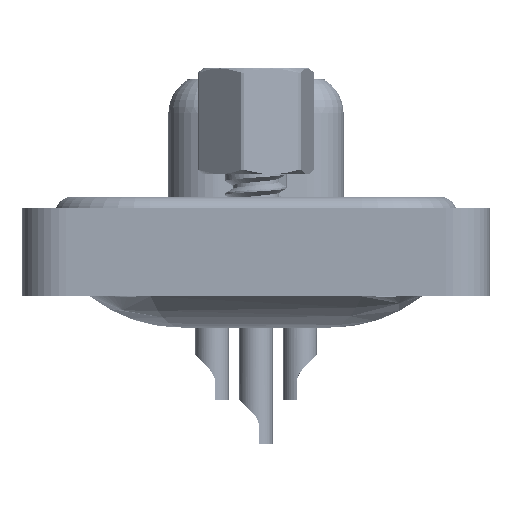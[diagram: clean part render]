
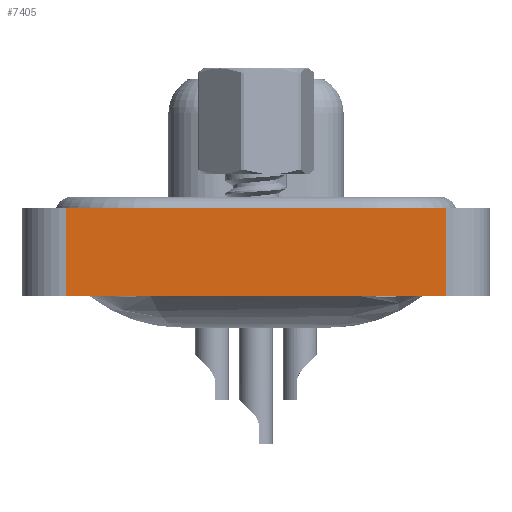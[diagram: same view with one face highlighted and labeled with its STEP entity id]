
A CAD part, left-side view. The second image highlights one B-rep face of the part: STEP entity #7405.
In plain terms, the highlighted planar face has unit normal (-1, 0, 0).
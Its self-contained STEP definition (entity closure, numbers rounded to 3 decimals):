
#681 = LINE ( 'NONE', #12842, #20764 ) ;
#2127 = ORIENTED_EDGE ( 'NONE', *, *, #33936, .T. ) ;
#3862 = DIRECTION ( 'NONE',  ( 0., 0., 1. ) ) ;
#6930 = ORIENTED_EDGE ( 'NONE', *, *, #33405, .F. ) ;
#7405 = ADVANCED_FACE ( 'NONE', ( #36830 ), #24727, .T. ) ;
#9623 = DIRECTION ( 'NONE',  ( -1., 0., 0. ) ) ;
#10217 = DIRECTION ( 'NONE',  ( 0., -1., 0. ) ) ;
#12154 = ORIENTED_EDGE ( 'NONE', *, *, #17473, .F. ) ;
#12842 = CARTESIAN_POINT ( 'NONE',  ( -7.35, 8.55, -3.6 ) ) ;
#12906 = EDGE_CURVE ( 'NONE', #13765, #13005, #27434, .T. ) ;
#13005 = VERTEX_POINT ( 'NONE', #34932 ) ;
#13195 = CARTESIAN_POINT ( 'NONE',  ( -7.35, -8.55, -3.6 ) ) ;
#13452 = CARTESIAN_POINT ( 'NONE',  ( -7.35, 8.55, -3.6 ) ) ;
#13703 = CARTESIAN_POINT ( 'NONE',  ( -7.35, -8.55, -3.6 ) ) ;
#13765 = VERTEX_POINT ( 'NONE', #29288 ) ;
#17473 = EDGE_CURVE ( 'NONE', #31483, #28309, #681, .T. ) ;
#19309 = AXIS2_PLACEMENT_3D ( 'NONE', #13195, #9623, #21757 ) ;
#19658 = DIRECTION ( 'NONE',  ( 0., -1., 0. ) ) ;
#20764 = VECTOR ( 'NONE', #3862, 1000. ) ;
#21757 = DIRECTION ( 'NONE',  ( 0., 0., 1. ) ) ;
#22054 = DIRECTION ( 'NONE',  ( 0., 0., 1. ) ) ;
#24727 = PLANE ( 'NONE',  #19309 ) ;
#25524 = CARTESIAN_POINT ( 'NONE',  ( -7.35, -8.55, 0.4 ) ) ;
#26589 = LINE ( 'NONE', #35723, #27261 ) ;
#27261 = VECTOR ( 'NONE', #19658, 1000. ) ;
#27434 = LINE ( 'NONE', #13703, #29465 ) ;
#28309 = VERTEX_POINT ( 'NONE', #31097 ) ;
#29288 = CARTESIAN_POINT ( 'NONE',  ( -7.35, -8.55, -3.6 ) ) ;
#29465 = VECTOR ( 'NONE', #22054, 1000. ) ;
#31097 = CARTESIAN_POINT ( 'NONE',  ( -7.35, 8.55, 0.4 ) ) ;
#31483 = VERTEX_POINT ( 'NONE', #13452 ) ;
#32251 = VECTOR ( 'NONE', #10217, 1000. ) ;
#33405 = EDGE_CURVE ( 'NONE', #28309, #13005, #35373, .T. ) ;
#33936 = EDGE_CURVE ( 'NONE', #31483, #13765, #26589, .T. ) ;
#34041 = EDGE_LOOP ( 'NONE', ( #36876, #6930, #12154, #2127 ) ) ;
#34932 = CARTESIAN_POINT ( 'NONE',  ( -7.35, -8.55, 0.4 ) ) ;
#35373 = LINE ( 'NONE', #25524, #32251 ) ;
#35723 = CARTESIAN_POINT ( 'NONE',  ( -7.35, -8.55, -3.6 ) ) ;
#36830 = FACE_OUTER_BOUND ( 'NONE', #34041, .T. ) ;
#36876 = ORIENTED_EDGE ( 'NONE', *, *, #12906, .T. ) ;
